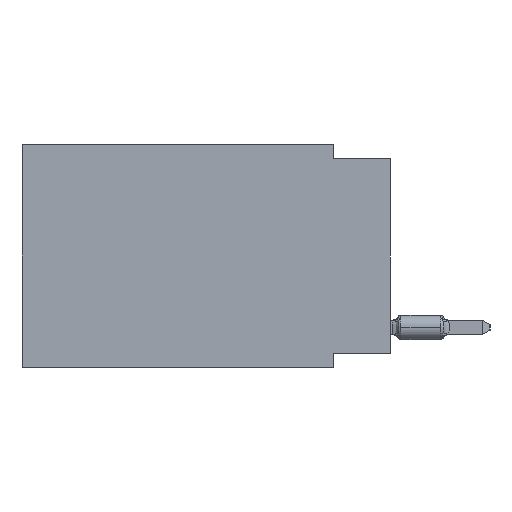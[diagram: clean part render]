
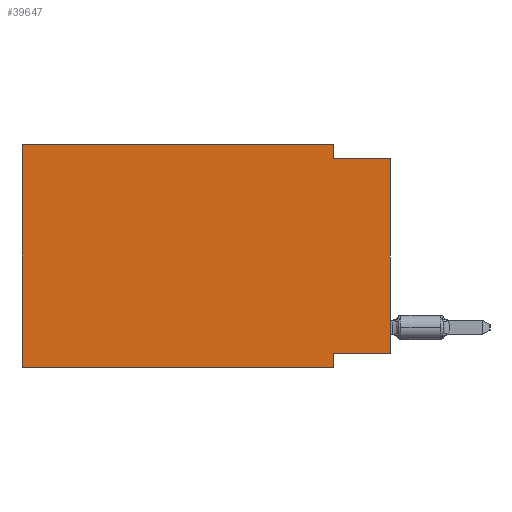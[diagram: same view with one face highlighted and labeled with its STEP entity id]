
A CAD part, left-side view. The second image highlights one B-rep face of the part: STEP entity #39647.
In plain terms, the highlighted planar face has unit normal (-1, 0, 0).
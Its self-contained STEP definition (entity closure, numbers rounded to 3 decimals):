
#206 = VERTEX_POINT ( 'NONE', #45987 ) ;
#746 = CARTESIAN_POINT ( 'NONE',  ( 0., 16.383, 0. ) ) ;
#1458 = VECTOR ( 'NONE', #41777, 1000. ) ;
#2399 = ORIENTED_EDGE ( 'NONE', *, *, #50102, .F. ) ;
#3253 = FACE_OUTER_BOUND ( 'NONE', #18964, .T. ) ;
#5134 = CARTESIAN_POINT ( 'NONE',  ( 0., 0., -0.635 ) ) ;
#6684 = CARTESIAN_POINT ( 'NONE',  ( 0., 0., -9.271 ) ) ;
#7189 = VERTEX_POINT ( 'NONE', #14637 ) ;
#7432 = EDGE_CURVE ( 'NONE', #206, #13728, #37182, .T. ) ;
#7448 = VERTEX_POINT ( 'NONE', #31868 ) ;
#8188 = CARTESIAN_POINT ( 'NONE',  ( 0., 16.383, -9.906 ) ) ;
#8593 = PLANE ( 'NONE',  #60851 ) ;
#9242 = VERTEX_POINT ( 'NONE', #24285 ) ;
#11053 = CARTESIAN_POINT ( 'NONE',  ( 0., 0., 0. ) ) ;
#13728 = VERTEX_POINT ( 'NONE', #28137 ) ;
#14467 = CARTESIAN_POINT ( 'NONE',  ( 0., 0., -0.635 ) ) ;
#14637 = CARTESIAN_POINT ( 'NONE',  ( 0., 2.54, -9.271 ) ) ;
#15830 = VERTEX_POINT ( 'NONE', #5134 ) ;
#16406 = VECTOR ( 'NONE', #49364, 1000. ) ;
#16537 = DIRECTION ( 'NONE',  ( 0., 0., 1. ) ) ;
#16772 = LINE ( 'NONE', #52423, #33674 ) ;
#16823 = EDGE_CURVE ( 'NONE', #13728, #15830, #57789, .T. ) ;
#18964 = EDGE_LOOP ( 'NONE', ( #56739, #54176, #59212, #22919, #2399, #31300, #27384, #40144 ) ) ;
#20625 = LINE ( 'NONE', #30984, #23635 ) ;
#22299 = LINE ( 'NONE', #8188, #1458 ) ;
#22919 = ORIENTED_EDGE ( 'NONE', *, *, #23541, .F. ) ;
#23541 = EDGE_CURVE ( 'NONE', #53103, #206, #30440, .T. ) ;
#23635 = VECTOR ( 'NONE', #16537, 1000. ) ;
#23800 = CARTESIAN_POINT ( 'NONE',  ( 0., 16.383, 0. ) ) ;
#24285 = CARTESIAN_POINT ( 'NONE',  ( 0., 0., -9.271 ) ) ;
#24944 = VECTOR ( 'NONE', #39941, 1000. ) ;
#26348 = CARTESIAN_POINT ( 'NONE',  ( 0., 2.54, -9.906 ) ) ;
#26882 = VECTOR ( 'NONE', #39242, 1000. ) ;
#27120 = CARTESIAN_POINT ( 'NONE',  ( 0., 16.383, 0. ) ) ;
#27384 = ORIENTED_EDGE ( 'NONE', *, *, #45756, .F. ) ;
#27424 = DIRECTION ( 'NONE',  ( 1., 0., 0. ) ) ;
#28137 = CARTESIAN_POINT ( 'NONE',  ( 0., 2.54, -0.635 ) ) ;
#30440 = LINE ( 'NONE', #746, #38436 ) ;
#30518 = LINE ( 'NONE', #11053, #24944 ) ;
#30984 = CARTESIAN_POINT ( 'NONE',  ( 0., 16.383, 0. ) ) ;
#31300 = ORIENTED_EDGE ( 'NONE', *, *, #35000, .T. ) ;
#31868 = CARTESIAN_POINT ( 'NONE',  ( 0., 16.383, -9.906 ) ) ;
#33674 = VECTOR ( 'NONE', #55069, 1000. ) ;
#35000 = EDGE_CURVE ( 'NONE', #7448, #50985, #22299, .T. ) ;
#37182 = LINE ( 'NONE', #56948, #51205 ) ;
#38436 = VECTOR ( 'NONE', #49585, 1000. ) ;
#39242 = DIRECTION ( 'NONE',  ( 0., -1., 0. ) ) ;
#39647 = ADVANCED_FACE ( 'NONE', ( #3253 ), #8593, .F. ) ;
#39941 = DIRECTION ( 'NONE',  ( 0., 0., 1. ) ) ;
#40144 = ORIENTED_EDGE ( 'NONE', *, *, #48376, .F. ) ;
#41777 = DIRECTION ( 'NONE',  ( 0., -1., 0. ) ) ;
#41888 = DIRECTION ( 'NONE',  ( 0., 0., -1. ) ) ;
#44346 = LINE ( 'NONE', #6684, #16406 ) ;
#45756 = EDGE_CURVE ( 'NONE', #7189, #50985, #16772, .T. ) ;
#45987 = CARTESIAN_POINT ( 'NONE',  ( 0., 2.54, 0. ) ) ;
#46265 = DIRECTION ( 'NONE',  ( 0., 0., -1. ) ) ;
#48376 = EDGE_CURVE ( 'NONE', #9242, #7189, #44346, .T. ) ;
#49364 = DIRECTION ( 'NONE',  ( 0., 1., 0. ) ) ;
#49585 = DIRECTION ( 'NONE',  ( 0., -1., 0. ) ) ;
#50102 = EDGE_CURVE ( 'NONE', #7448, #53103, #20625, .T. ) ;
#50985 = VERTEX_POINT ( 'NONE', #26348 ) ;
#51205 = VECTOR ( 'NONE', #41888, 1000. ) ;
#52423 = CARTESIAN_POINT ( 'NONE',  ( 0., 2.54, -9.906 ) ) ;
#53103 = VERTEX_POINT ( 'NONE', #23800 ) ;
#53599 = EDGE_CURVE ( 'NONE', #9242, #15830, #30518, .T. ) ;
#54176 = ORIENTED_EDGE ( 'NONE', *, *, #16823, .F. ) ;
#55069 = DIRECTION ( 'NONE',  ( 0., 0., -1. ) ) ;
#56739 = ORIENTED_EDGE ( 'NONE', *, *, #53599, .T. ) ;
#56948 = CARTESIAN_POINT ( 'NONE',  ( 0., 2.54, 0. ) ) ;
#57789 = LINE ( 'NONE', #14467, #26882 ) ;
#59212 = ORIENTED_EDGE ( 'NONE', *, *, #7432, .F. ) ;
#60851 = AXIS2_PLACEMENT_3D ( 'NONE', #27120, #27424, #46265 ) ;
